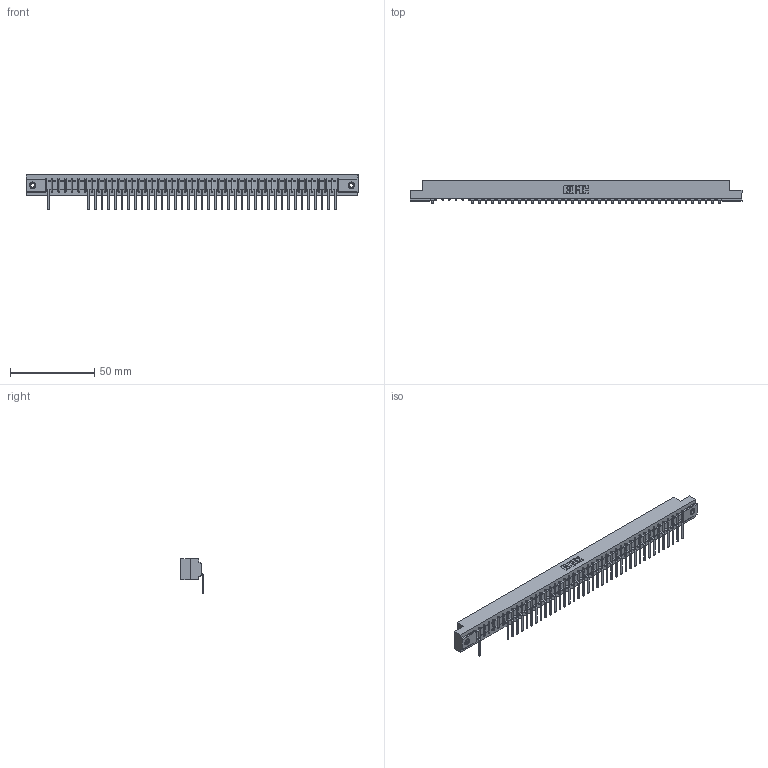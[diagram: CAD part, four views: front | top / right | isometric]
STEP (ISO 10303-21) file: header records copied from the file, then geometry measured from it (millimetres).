
FILE_DESCRIPTION (( 'STEP AP203' ), '1' );
FILE_NAME ('357-044-557-108.STEP', '2018-08-11T11:52:56', ( '' ), ( '' ), 'SwSTEP 2.0', 'SolidWorks 2016', '' );
FILE_SCHEMA (( 'CONFIG_CONTROL_DESIGN' ));
Length unit declared in the file: inch
Products named in the file (4): 307 Part_.156 Dia Mounting Holes; 307-290-002_557; 345-250-001_345-250-003-102; 357-044-557-108
Assembly tree (42 placements, depth 2):
  357-044-557-108
    307 Part_.156 Dia Mounting Holes
    307-290-002_557  x39
    345-250-001_345-250-003-102  x2
Bounding box: 197.36 x 13.32 x 20.66 mm (x, y, z)
Volume: 21088.8 mm3; surface area: 26336.7 mm2
Topology: 42 solids, 42 shells, 3365 faces, 10295 edges, 6734 vertices
Faces by surface type: plane 1995, cylinder 1264, sphere 90, cone 12, torus 4
Entity records: 39353 total; most frequent: CARTESIAN_POINT 6642, ORIENTED_EDGE 6630, DIRECTION 6457, EDGE_CURVE 3315, VECTOR 2539, LINE 2539, VERTEX_POINT 2144, AXIS2_PLACEMENT_3D 1959
